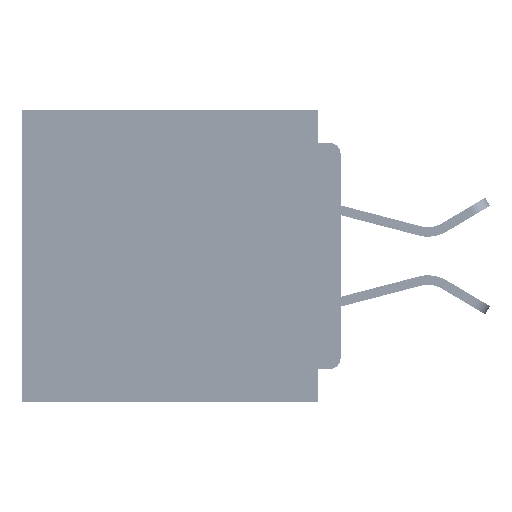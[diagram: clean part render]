
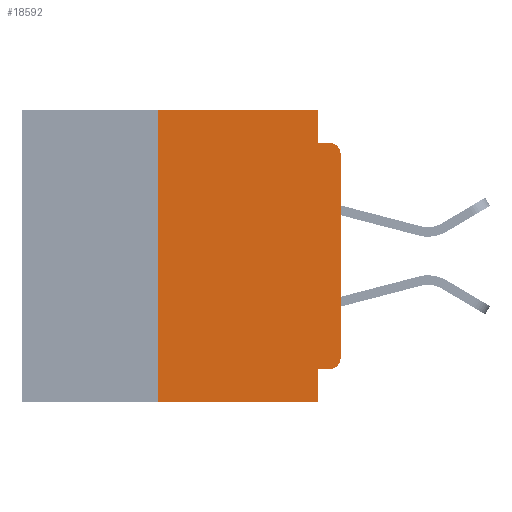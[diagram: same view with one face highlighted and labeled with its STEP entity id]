
A CAD part, left-side view. The second image highlights one B-rep face of the part: STEP entity #18592.
In plain terms, the highlighted planar face has unit normal (-1, 0, 0).
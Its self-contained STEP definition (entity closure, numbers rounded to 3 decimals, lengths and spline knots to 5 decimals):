
#90 = CARTESIAN_POINT ( 'NONE',  ( 0., 0.031, -0.355 ) ) ;
#284 = CARTESIAN_POINT ( 'NONE',  ( 0., 0.437, 0. ) ) ;
#420 = VERTEX_POINT ( 'NONE', #45985 ) ;
#1574 = CARTESIAN_POINT ( 'NONE',  ( 0., 0.437, 0. ) ) ;
#1776 = CARTESIAN_POINT ( 'NONE',  ( 0., 0., 0. ) ) ;
#2281 = EDGE_CURVE ( 'NONE', #7544, #42849, #49562, .T. ) ;
#2851 = VECTOR ( 'NONE', #45718, 39.37008 ) ;
#3128 = ORIENTED_EDGE ( 'NONE', *, *, #47487, .F. ) ;
#3717 = EDGE_CURVE ( 'NONE', #420, #48508, #19467, .T. ) ;
#4486 = LINE ( 'NONE', #8983, #15699 ) ;
#4667 = DIRECTION ( 'NONE',  ( 0., 0., -1. ) ) ;
#4734 = CARTESIAN_POINT ( 'NONE',  ( 0., 0.031, -0.4 ) ) ;
#5783 = DIRECTION ( 'NONE',  ( 0., -1., 0. ) ) ;
#6200 = CARTESIAN_POINT ( 'NONE',  ( 0., 0.015, -0.06 ) ) ;
#6507 = LINE ( 'NONE', #4734, #34048 ) ;
#7118 = DIRECTION ( 'NONE',  ( 1., 0., 0. ) ) ;
#7544 = VERTEX_POINT ( 'NONE', #49164 ) ;
#7666 = EDGE_CURVE ( 'NONE', #61948, #14763, #29479, .T. ) ;
#8983 = CARTESIAN_POINT ( 'NONE',  ( 0., 0., -0.045 ) ) ;
#11628 = EDGE_CURVE ( 'NONE', #13415, #36746, #69154, .T. ) ;
#11766 = DIRECTION ( 'NONE',  ( 0., 0., -1. ) ) ;
#12101 = VERTEX_POINT ( 'NONE', #31480 ) ;
#12592 = VECTOR ( 'NONE', #52732, 39.37008 ) ;
#12688 = EDGE_CURVE ( 'NONE', #13415, #12101, #70939, .T. ) ;
#13415 = VERTEX_POINT ( 'NONE', #53794 ) ;
#14367 = EDGE_CURVE ( 'NONE', #65045, #61948, #17503, .T. ) ;
#14397 = CARTESIAN_POINT ( 'NONE',  ( 0., 0.031, -0.4 ) ) ;
#14763 = VERTEX_POINT ( 'NONE', #22443 ) ;
#15699 = VECTOR ( 'NONE', #41871, 39.37008 ) ;
#16054 = DIRECTION ( 'NONE',  ( 0., 0., -1. ) ) ;
#17503 = LINE ( 'NONE', #1776, #2851 ) ;
#17532 = DIRECTION ( 'NONE',  ( 0., 1., 0. ) ) ;
#18592 = ADVANCED_FACE ( 'NONE', ( #47279 ), #67316, .F. ) ;
#19423 = CARTESIAN_POINT ( 'NONE',  ( 0., 0., -0.355 ) ) ;
#19467 = LINE ( 'NONE', #46117, #59818 ) ;
#21236 = EDGE_CURVE ( 'NONE', #42849, #36746, #6507, .T. ) ;
#21708 = CARTESIAN_POINT ( 'NONE',  ( 0., 0.437, -0.4 ) ) ;
#22443 = CARTESIAN_POINT ( 'NONE',  ( 0., 0.015, -0.045 ) ) ;
#24745 = CARTESIAN_POINT ( 'NONE',  ( 0., 0., -0.06 ) ) ;
#25555 = EDGE_CURVE ( 'NONE', #7544, #65045, #55358, .T. ) ;
#29479 = CIRCLE ( 'NONE', #57555, 0.015 ) ;
#30578 = VECTOR ( 'NONE', #54578, 39.37008 ) ;
#31480 = CARTESIAN_POINT ( 'NONE',  ( 0., 0.25, 0. ) ) ;
#31737 = CARTESIAN_POINT ( 'NONE',  ( 0., 0.031, -0.045 ) ) ;
#33612 = VECTOR ( 'NONE', #5783, 39.37008 ) ;
#33940 = ORIENTED_EDGE ( 'NONE', *, *, #14367, .T. ) ;
#34048 = VECTOR ( 'NONE', #16054, 39.37008 ) ;
#35027 = VECTOR ( 'NONE', #17532, 39.37008 ) ;
#35454 = EDGE_LOOP ( 'NONE', ( #33940, #69861, #36880, #61488, #3128, #61970, #60702, #51785, #42842, #63041 ) ) ;
#36746 = VERTEX_POINT ( 'NONE', #14397 ) ;
#36880 = ORIENTED_EDGE ( 'NONE', *, *, #49721, .F. ) ;
#37626 = DIRECTION ( 'NONE',  ( -1., 0., 0. ) ) ;
#41871 = DIRECTION ( 'NONE',  ( 0., -1., 0. ) ) ;
#42842 = ORIENTED_EDGE ( 'NONE', *, *, #2281, .F. ) ;
#42849 = VERTEX_POINT ( 'NONE', #90 ) ;
#44657 = DIRECTION ( 'NONE',  ( -1., 0., 0. ) ) ;
#45537 = DIRECTION ( 'NONE',  ( 0., 0., -1. ) ) ;
#45718 = DIRECTION ( 'NONE',  ( 0., 0., 1. ) ) ;
#45840 = DIRECTION ( 'NONE',  ( 0., 0., -1. ) ) ;
#45985 = CARTESIAN_POINT ( 'NONE',  ( 0., 0.031, 0. ) ) ;
#46117 = CARTESIAN_POINT ( 'NONE',  ( 0., 0.031, 0. ) ) ;
#47201 = CARTESIAN_POINT ( 'NONE',  ( 0., 0.25, -0.4 ) ) ;
#47279 = FACE_OUTER_BOUND ( 'NONE', #35454, .T. ) ;
#47487 = EDGE_CURVE ( 'NONE', #12101, #420, #62756, .T. ) ;
#48508 = VERTEX_POINT ( 'NONE', #31737 ) ;
#49164 = CARTESIAN_POINT ( 'NONE',  ( 0., 0.015, -0.355 ) ) ;
#49562 = LINE ( 'NONE', #19423, #35027 ) ;
#49721 = EDGE_CURVE ( 'NONE', #48508, #14763, #4486, .T. ) ;
#51785 = ORIENTED_EDGE ( 'NONE', *, *, #21236, .F. ) ;
#52732 = DIRECTION ( 'NONE',  ( 0., 0., 1. ) ) ;
#53794 = CARTESIAN_POINT ( 'NONE',  ( 0., 0.25, -0.4 ) ) ;
#54578 = DIRECTION ( 'NONE',  ( 0., -1., 0. ) ) ;
#55303 = AXIS2_PLACEMENT_3D ( 'NONE', #70427, #37626, #4667 ) ;
#55358 = CIRCLE ( 'NONE', #55303, 0.015 ) ;
#57555 = AXIS2_PLACEMENT_3D ( 'NONE', #6200, #44657, #11766 ) ;
#59818 = VECTOR ( 'NONE', #45840, 39.37008 ) ;
#60604 = CARTESIAN_POINT ( 'NONE',  ( 0., 0., -0.34 ) ) ;
#60702 = ORIENTED_EDGE ( 'NONE', *, *, #11628, .T. ) ;
#61488 = ORIENTED_EDGE ( 'NONE', *, *, #3717, .F. ) ;
#61948 = VERTEX_POINT ( 'NONE', #24745 ) ;
#61970 = ORIENTED_EDGE ( 'NONE', *, *, #12688, .F. ) ;
#62756 = LINE ( 'NONE', #284, #33612 ) ;
#63041 = ORIENTED_EDGE ( 'NONE', *, *, #25555, .T. ) ;
#64608 = AXIS2_PLACEMENT_3D ( 'NONE', #1574, #7118, #45537 ) ;
#65045 = VERTEX_POINT ( 'NONE', #60604 ) ;
#67316 = PLANE ( 'NONE',  #64608 ) ;
#69154 = LINE ( 'NONE', #21708, #30578 ) ;
#69861 = ORIENTED_EDGE ( 'NONE', *, *, #7666, .T. ) ;
#70427 = CARTESIAN_POINT ( 'NONE',  ( 0., 0.015, -0.34 ) ) ;
#70939 = LINE ( 'NONE', #47201, #12592 ) ;
